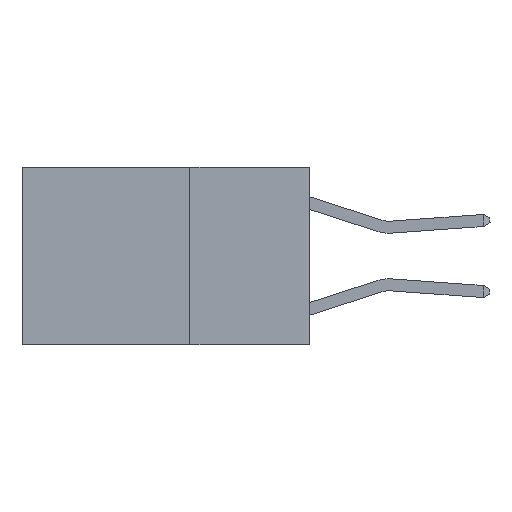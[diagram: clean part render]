
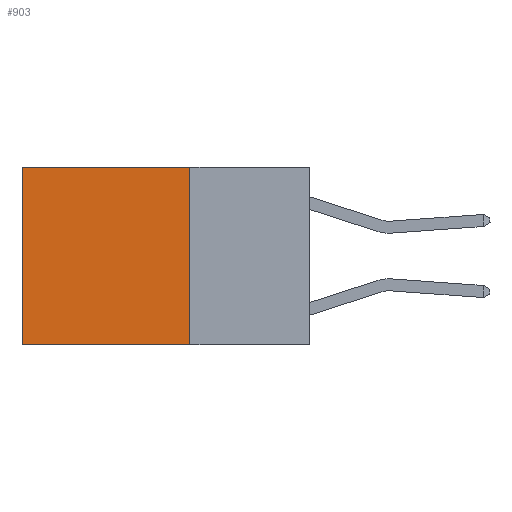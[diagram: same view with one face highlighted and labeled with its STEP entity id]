
A CAD part, left-side view. The second image highlights one B-rep face of the part: STEP entity #903.
In plain terms, the highlighted planar face has unit normal (-1, 0, 0).
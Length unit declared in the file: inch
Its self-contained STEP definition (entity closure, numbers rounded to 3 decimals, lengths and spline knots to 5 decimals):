
#139 = CARTESIAN_POINT ( 'NONE',  ( 0.2625, 0.25, 0. ) ) ;
#477 = CARTESIAN_POINT ( 'NONE',  ( 0.2625, 0.6, 0. ) ) ;
#648 = VECTOR ( 'NONE', #1347, 39.37008 ) ;
#722 = LINE ( 'NONE', #5781, #7799 ) ;
#903 = ADVANCED_FACE ( 'NONE', ( #4674 ), #3199, .F. ) ;
#1091 = EDGE_LOOP ( 'NONE', ( #1641, #1527, #2607, #5577 ) ) ;
#1226 = VERTEX_POINT ( 'NONE', #8529 ) ;
#1347 = DIRECTION ( 'NONE',  ( 0., 0., -1. ) ) ;
#1480 = EDGE_CURVE ( 'NONE', #6119, #1226, #5308, .T. ) ;
#1527 = ORIENTED_EDGE ( 'NONE', *, *, #2883, .F. ) ;
#1632 = VERTEX_POINT ( 'NONE', #7010 ) ;
#1641 = ORIENTED_EDGE ( 'NONE', *, *, #2285, .T. ) ;
#2285 = EDGE_CURVE ( 'NONE', #1226, #4648, #7958, .T. ) ;
#2607 = ORIENTED_EDGE ( 'NONE', *, *, #5971, .F. ) ;
#2766 = LINE ( 'NONE', #3396, #4403 ) ;
#2883 = EDGE_CURVE ( 'NONE', #1632, #4648, #2766, .T. ) ;
#3199 = PLANE ( 'NONE',  #8254 ) ;
#3396 = CARTESIAN_POINT ( 'NONE',  ( 0.2625, 0.25, -0.37 ) ) ;
#3421 = VECTOR ( 'NONE', #5430, 39.37008 ) ;
#3887 = DIRECTION ( 'NONE',  ( 1., 0., 0. ) ) ;
#3993 = CARTESIAN_POINT ( 'NONE',  ( 0.2625, 0.25, 0. ) ) ;
#4403 = VECTOR ( 'NONE', #6246, 39.37008 ) ;
#4648 = VERTEX_POINT ( 'NONE', #5182 ) ;
#4674 = FACE_OUTER_BOUND ( 'NONE', #1091, .T. ) ;
#5182 = CARTESIAN_POINT ( 'NONE',  ( 0.2625, 0.6, -0.37 ) ) ;
#5308 = LINE ( 'NONE', #3993, #3421 ) ;
#5430 = DIRECTION ( 'NONE',  ( 0., 1., 0. ) ) ;
#5577 = ORIENTED_EDGE ( 'NONE', *, *, #1480, .T. ) ;
#5583 = CARTESIAN_POINT ( 'NONE',  ( 0.2625, 0.25, 0. ) ) ;
#5781 = CARTESIAN_POINT ( 'NONE',  ( 0.2625, 0.25, 0. ) ) ;
#5971 = EDGE_CURVE ( 'NONE', #6119, #1632, #722, .T. ) ;
#6119 = VERTEX_POINT ( 'NONE', #5583 ) ;
#6246 = DIRECTION ( 'NONE',  ( 0., 1., 0. ) ) ;
#6479 = DIRECTION ( 'NONE',  ( 0., 0., -1. ) ) ;
#7010 = CARTESIAN_POINT ( 'NONE',  ( 0.2625, 0.25, -0.37 ) ) ;
#7799 = VECTOR ( 'NONE', #6479, 39.37008 ) ;
#7958 = LINE ( 'NONE', #477, #648 ) ;
#8254 = AXIS2_PLACEMENT_3D ( 'NONE', #139, #3887, #8702 ) ;
#8529 = CARTESIAN_POINT ( 'NONE',  ( 0.2625, 0.6, 0. ) ) ;
#8702 = DIRECTION ( 'NONE',  ( 0., 0., -1. ) ) ;
